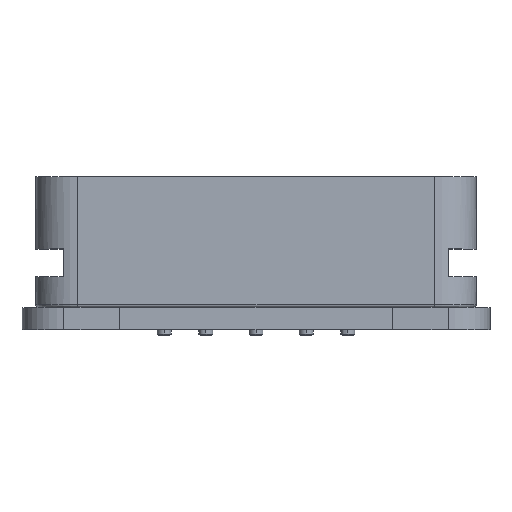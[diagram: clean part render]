
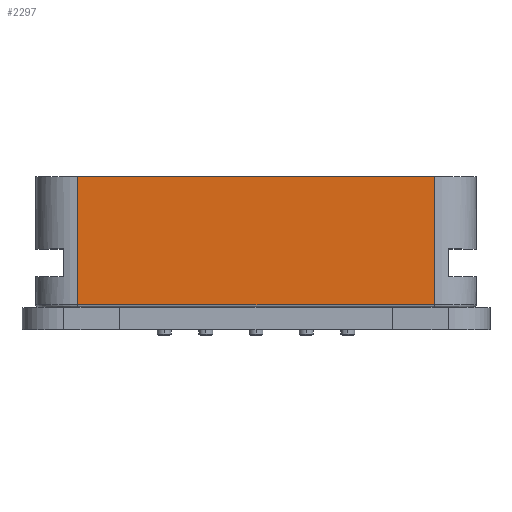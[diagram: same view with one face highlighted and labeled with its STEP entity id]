
A CAD part, top view. The second image highlights one B-rep face of the part: STEP entity #2297.
In plain terms, the highlighted planar face has unit normal (0, 0, 1).
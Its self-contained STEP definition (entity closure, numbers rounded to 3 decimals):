
#127 = EDGE_CURVE ( 'NONE', #3206, #307, #2986, .T. ) ;
#193 = DIRECTION ( 'NONE',  ( 0., 0., -1. ) ) ;
#249 = VECTOR ( 'NONE', #2906, 1000. ) ;
#307 = VERTEX_POINT ( 'NONE', #1957 ) ;
#455 = DIRECTION ( 'NONE',  ( 1., 0., 0. ) ) ;
#521 = EDGE_CURVE ( 'NONE', #3206, #3554, #2670, .T. ) ;
#596 = VECTOR ( 'NONE', #2426, 1000. ) ;
#678 = CARTESIAN_POINT ( 'NONE',  ( 6.4, 4.7, 2.1 ) ) ;
#977 = LINE ( 'NONE', #678, #249 ) ;
#1083 = CARTESIAN_POINT ( 'NONE',  ( -6.4, 4.7, 2.1 ) ) ;
#1214 = VERTEX_POINT ( 'NONE', #2807 ) ;
#1220 = EDGE_LOOP ( 'NONE', ( #2066, #1461, #1278, #2466 ) ) ;
#1248 = CARTESIAN_POINT ( 'NONE',  ( -6.4, 0.1, 2.1 ) ) ;
#1278 = ORIENTED_EDGE ( 'NONE', *, *, #521, .T. ) ;
#1461 = ORIENTED_EDGE ( 'NONE', *, *, #127, .F. ) ;
#1815 = DIRECTION ( 'NONE',  ( 0., -1., 0. ) ) ;
#1820 = CARTESIAN_POINT ( 'NONE',  ( -6.4, 4.7, 2.1 ) ) ;
#1957 = CARTESIAN_POINT ( 'NONE',  ( 6.4, 4.7, 2.1 ) ) ;
#2066 = ORIENTED_EDGE ( 'NONE', *, *, #2645, .F. ) ;
#2085 = CARTESIAN_POINT ( 'NONE',  ( -6.4, 4.7, 2.1 ) ) ;
#2126 = CARTESIAN_POINT ( 'NONE',  ( -6.4, 4.7, 2.1 ) ) ;
#2200 = VECTOR ( 'NONE', #455, 1000. ) ;
#2259 = AXIS2_PLACEMENT_3D ( 'NONE', #1083, #193, #3325 ) ;
#2297 = ADVANCED_FACE ( 'NONE', ( #2451 ), #3309, .F. ) ;
#2426 = DIRECTION ( 'NONE',  ( 1., 0., 0. ) ) ;
#2451 = FACE_OUTER_BOUND ( 'NONE', #1220, .T. ) ;
#2466 = ORIENTED_EDGE ( 'NONE', *, *, #2711, .T. ) ;
#2645 = EDGE_CURVE ( 'NONE', #307, #1214, #977, .T. ) ;
#2670 = LINE ( 'NONE', #2126, #3643 ) ;
#2711 = EDGE_CURVE ( 'NONE', #3554, #1214, #3005, .T. ) ;
#2807 = CARTESIAN_POINT ( 'NONE',  ( 6.4, 0.1, 2.1 ) ) ;
#2906 = DIRECTION ( 'NONE',  ( 0., -1., 0. ) ) ;
#2986 = LINE ( 'NONE', #1820, #596 ) ;
#3005 = LINE ( 'NONE', #3579, #2200 ) ;
#3206 = VERTEX_POINT ( 'NONE', #2085 ) ;
#3309 = PLANE ( 'NONE',  #2259 ) ;
#3325 = DIRECTION ( 'NONE',  ( -1., 0., 0. ) ) ;
#3554 = VERTEX_POINT ( 'NONE', #1248 ) ;
#3579 = CARTESIAN_POINT ( 'NONE',  ( 6.4, 0.1, 2.1 ) ) ;
#3643 = VECTOR ( 'NONE', #1815, 1000. ) ;
